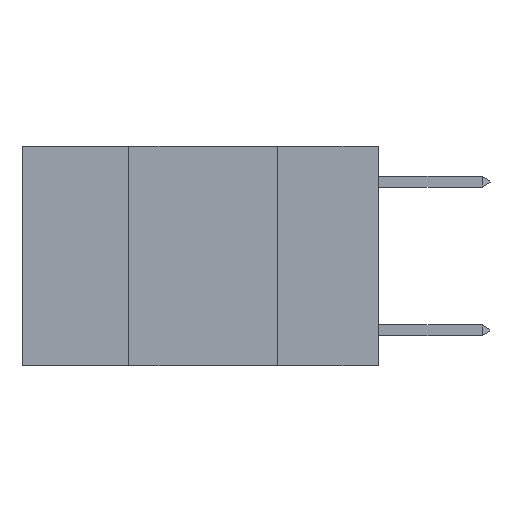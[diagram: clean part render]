
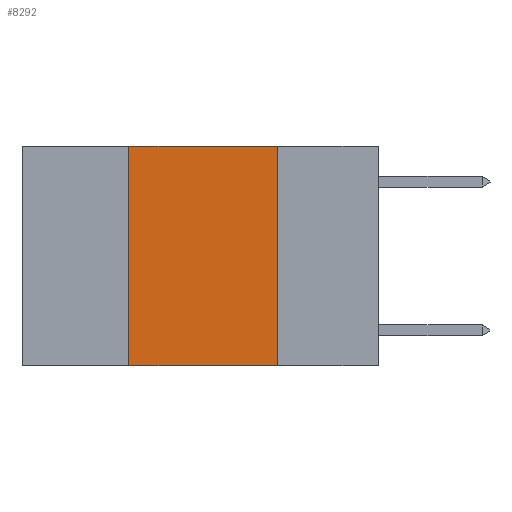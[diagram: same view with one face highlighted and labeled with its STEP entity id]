
A CAD part, left-side view. The second image highlights one B-rep face of the part: STEP entity #8292.
In plain terms, the highlighted planar face has unit normal (-1, 0, 0).
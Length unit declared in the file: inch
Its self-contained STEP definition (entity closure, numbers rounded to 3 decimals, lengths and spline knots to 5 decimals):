
#435 = EDGE_CURVE ( 'NONE', #3932, #5733, #8106, .T. ) ;
#584 = EDGE_CURVE ( 'NONE', #5733, #3947, #652, .T. ) ;
#652 = LINE ( 'NONE', #3270, #5719 ) ;
#682 = DIRECTION ( 'NONE',  ( 1., 0., 0. ) ) ;
#695 = DIRECTION ( 'NONE',  ( 0., 0., -1. ) ) ;
#800 = LINE ( 'NONE', #6064, #7036 ) ;
#2716 = DIRECTION ( 'NONE',  ( 0., -1., 0. ) ) ;
#2777 = CARTESIAN_POINT ( 'NONE',  ( 0., 0.42, 0. ) ) ;
#2827 = VECTOR ( 'NONE', #3585, 39.37008 ) ;
#2916 = ORIENTED_EDGE ( 'NONE', *, *, #3426, .T. ) ;
#3270 = CARTESIAN_POINT ( 'NONE',  ( 0., 0.17, 0. ) ) ;
#3426 = EDGE_CURVE ( 'NONE', #4374, #3947, #800, .T. ) ;
#3469 = VECTOR ( 'NONE', #7135, 39.37008 ) ;
#3585 = DIRECTION ( 'NONE',  ( 0., -1., 0. ) ) ;
#3812 = EDGE_CURVE ( 'NONE', #4374, #3932, #6549, .T. ) ;
#3858 = ORIENTED_EDGE ( 'NONE', *, *, #435, .F. ) ;
#3932 = VERTEX_POINT ( 'NONE', #2777 ) ;
#3947 = VERTEX_POINT ( 'NONE', #8089 ) ;
#4374 = VERTEX_POINT ( 'NONE', #7959 ) ;
#4512 = ORIENTED_EDGE ( 'NONE', *, *, #584, .F. ) ;
#4547 = DIRECTION ( 'NONE',  ( 0., 0., -1. ) ) ;
#4595 = PLANE ( 'NONE',  #7732 ) ;
#5477 = EDGE_LOOP ( 'NONE', ( #4512, #3858, #6850, #2916 ) ) ;
#5681 = CARTESIAN_POINT ( 'NONE',  ( 0., 0.6, 0. ) ) ;
#5719 = VECTOR ( 'NONE', #695, 39.37008 ) ;
#5733 = VERTEX_POINT ( 'NONE', #7420 ) ;
#5843 = CARTESIAN_POINT ( 'NONE',  ( 0., 0.6, 0. ) ) ;
#6064 = CARTESIAN_POINT ( 'NONE',  ( 0., 0.6, -0.37 ) ) ;
#6549 = LINE ( 'NONE', #7804, #3469 ) ;
#6850 = ORIENTED_EDGE ( 'NONE', *, *, #3812, .F. ) ;
#7036 = VECTOR ( 'NONE', #2716, 39.37008 ) ;
#7135 = DIRECTION ( 'NONE',  ( 0., 0., 1. ) ) ;
#7420 = CARTESIAN_POINT ( 'NONE',  ( 0., 0.17, 0. ) ) ;
#7732 = AXIS2_PLACEMENT_3D ( 'NONE', #5843, #682, #4547 ) ;
#7804 = CARTESIAN_POINT ( 'NONE',  ( 0., 0.42, 0. ) ) ;
#7948 = FACE_OUTER_BOUND ( 'NONE', #5477, .T. ) ;
#7959 = CARTESIAN_POINT ( 'NONE',  ( 0., 0.42, -0.37 ) ) ;
#8089 = CARTESIAN_POINT ( 'NONE',  ( 0., 0.17, -0.37 ) ) ;
#8106 = LINE ( 'NONE', #5681, #2827 ) ;
#8292 = ADVANCED_FACE ( 'NONE', ( #7948 ), #4595, .F. ) ;
